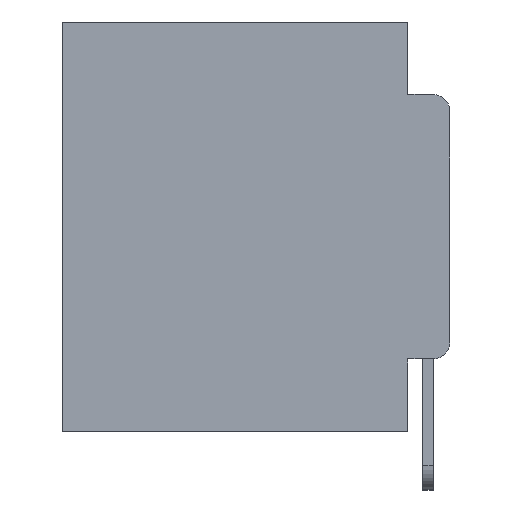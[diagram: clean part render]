
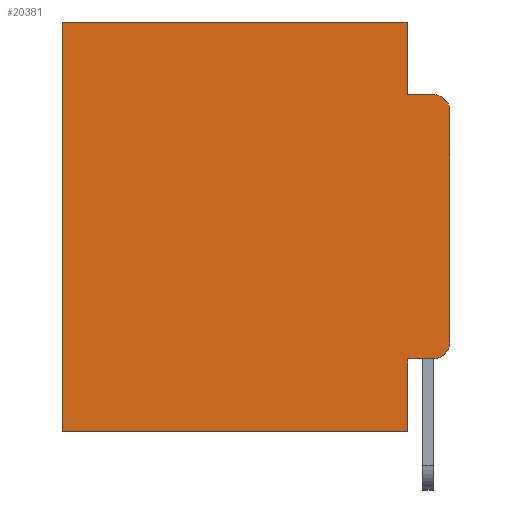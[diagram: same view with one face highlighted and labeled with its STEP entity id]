
A CAD part, left-side view. The second image highlights one B-rep face of the part: STEP entity #20381.
In plain terms, the highlighted planar face has unit normal (-1, 0, 0).
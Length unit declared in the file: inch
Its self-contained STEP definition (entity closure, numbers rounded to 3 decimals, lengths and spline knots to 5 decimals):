
#599 = VERTEX_POINT ( 'NONE', #14311 ) ;
#816 = VECTOR ( 'NONE', #19525, 39.37008 ) ;
#961 = CIRCLE ( 'NONE', #5620, 0.02 ) ;
#1031 = CARTESIAN_POINT ( 'NONE',  ( 0.298, 0., -0.5 ) ) ;
#1295 = DIRECTION ( 'NONE',  ( -1., 0., 0. ) ) ;
#1548 = AXIS2_PLACEMENT_3D ( 'NONE', #20681, #10157, #25126 ) ;
#1671 = CARTESIAN_POINT ( 'NONE',  ( 0.298, 0.051, 0. ) ) ;
#1893 = DIRECTION ( 'NONE',  ( 0., -1., 0. ) ) ;
#1897 = LINE ( 'NONE', #18239, #16613 ) ;
#2006 = LINE ( 'NONE', #21167, #19800 ) ;
#3149 = PLANE ( 'NONE',  #22982 ) ;
#3543 = LINE ( 'NONE', #19341, #816 ) ;
#3923 = EDGE_CURVE ( 'NONE', #20177, #22243, #6880, .T. ) ;
#4136 = VECTOR ( 'NONE', #6309, 39.37008 ) ;
#4221 = EDGE_CURVE ( 'NONE', #23742, #18434, #1897, .T. ) ;
#4287 = ORIENTED_EDGE ( 'NONE', *, *, #14657, .F. ) ;
#4483 = ORIENTED_EDGE ( 'NONE', *, *, #4221, .F. ) ;
#5059 = EDGE_CURVE ( 'NONE', #19185, #599, #14233, .T. ) ;
#5294 = DIRECTION ( 'NONE',  ( 0., 0., -1. ) ) ;
#5332 = DIRECTION ( 'NONE',  ( 0., 0., -1. ) ) ;
#5620 = AXIS2_PLACEMENT_3D ( 'NONE', #16380, #1295, #5332 ) ;
#6309 = DIRECTION ( 'NONE',  ( 0., 1., 0. ) ) ;
#6621 = CARTESIAN_POINT ( 'NONE',  ( 0.298, 0.473, 0. ) ) ;
#6880 = LINE ( 'NONE', #1671, #7564 ) ;
#7354 = FACE_OUTER_BOUND ( 'NONE', #10778, .T. ) ;
#7564 = VECTOR ( 'NONE', #12456, 39.37008 ) ;
#7922 = CIRCLE ( 'NONE', #1548, 0.02 ) ;
#8072 = CARTESIAN_POINT ( 'NONE',  ( 0.298, 0., -0.1085 ) ) ;
#8854 = VECTOR ( 'NONE', #9164, 39.37008 ) ;
#9157 = ORIENTED_EDGE ( 'NONE', *, *, #12754, .F. ) ;
#9164 = DIRECTION ( 'NONE',  ( 0., 0., -1. ) ) ;
#9547 = CARTESIAN_POINT ( 'NONE',  ( 0.298, 0.473, 0. ) ) ;
#10157 = DIRECTION ( 'NONE',  ( -1., 0., 0. ) ) ;
#10434 = VERTEX_POINT ( 'NONE', #8072 ) ;
#10778 = EDGE_LOOP ( 'NONE', ( #4287, #15771, #27266, #4483, #14500, #23023, #9157, #10780, #11809, #15659 ) ) ;
#10780 = ORIENTED_EDGE ( 'NONE', *, *, #3923, .F. ) ;
#11809 = ORIENTED_EDGE ( 'NONE', *, *, #18355, .T. ) ;
#11925 = CARTESIAN_POINT ( 'NONE',  ( 0.298, 0.051, -0.4115 ) ) ;
#12294 = VERTEX_POINT ( 'NONE', #17871 ) ;
#12456 = DIRECTION ( 'NONE',  ( 0., 0., -1. ) ) ;
#12754 = EDGE_CURVE ( 'NONE', #22243, #599, #23510, .T. ) ;
#13757 = CARTESIAN_POINT ( 'NONE',  ( 0.298, 0.02, -0.0885 ) ) ;
#13914 = DIRECTION ( 'NONE',  ( 0., 0., -1. ) ) ;
#14103 = CARTESIAN_POINT ( 'NONE',  ( 0.298, 0.051, -0.5 ) ) ;
#14233 = LINE ( 'NONE', #9547, #8854 ) ;
#14311 = CARTESIAN_POINT ( 'NONE',  ( 0.298, 0.473, -0.5 ) ) ;
#14441 = VERTEX_POINT ( 'NONE', #16406 ) ;
#14500 = ORIENTED_EDGE ( 'NONE', *, *, #16170, .T. ) ;
#14657 = EDGE_CURVE ( 'NONE', #10434, #14441, #3543, .T. ) ;
#15659 = ORIENTED_EDGE ( 'NONE', *, *, #22932, .T. ) ;
#15771 = ORIENTED_EDGE ( 'NONE', *, *, #18776, .T. ) ;
#16170 = EDGE_CURVE ( 'NONE', #23742, #19185, #16871, .T. ) ;
#16380 = CARTESIAN_POINT ( 'NONE',  ( 0.298, 0.02, -0.1085 ) ) ;
#16406 = CARTESIAN_POINT ( 'NONE',  ( 0.298, 0., -0.3915 ) ) ;
#16613 = VECTOR ( 'NONE', #5294, 39.37008 ) ;
#16871 = LINE ( 'NONE', #16974, #4136 ) ;
#16974 = CARTESIAN_POINT ( 'NONE',  ( 0.298, 0., 0. ) ) ;
#17205 = EDGE_CURVE ( 'NONE', #18434, #25533, #24944, .T. ) ;
#17255 = CARTESIAN_POINT ( 'NONE',  ( 0.298, 0.051, -0.0885 ) ) ;
#17395 = VECTOR ( 'NONE', #18205, 39.37008 ) ;
#17871 = CARTESIAN_POINT ( 'NONE',  ( 0.298, 0.02, -0.4115 ) ) ;
#18151 = DIRECTION ( 'NONE',  ( 1., 0., 0. ) ) ;
#18205 = DIRECTION ( 'NONE',  ( 0., 1., 0. ) ) ;
#18239 = CARTESIAN_POINT ( 'NONE',  ( 0.298, 0.051, 0. ) ) ;
#18355 = EDGE_CURVE ( 'NONE', #20177, #12294, #2006, .T. ) ;
#18434 = VERTEX_POINT ( 'NONE', #17255 ) ;
#18776 = EDGE_CURVE ( 'NONE', #10434, #25533, #961, .T. ) ;
#19185 = VERTEX_POINT ( 'NONE', #6621 ) ;
#19341 = CARTESIAN_POINT ( 'NONE',  ( 0.298, 0., 0. ) ) ;
#19525 = DIRECTION ( 'NONE',  ( 0., 0., -1. ) ) ;
#19800 = VECTOR ( 'NONE', #1893, 39.37008 ) ;
#19865 = DIRECTION ( 'NONE',  ( 0., -1., 0. ) ) ;
#20177 = VERTEX_POINT ( 'NONE', #11925 ) ;
#20381 = ADVANCED_FACE ( 'NONE', ( #7354 ), #3149, .F. ) ;
#20681 = CARTESIAN_POINT ( 'NONE',  ( 0.298, 0.02, -0.3915 ) ) ;
#21167 = CARTESIAN_POINT ( 'NONE',  ( 0.298, 0.051, -0.4115 ) ) ;
#22145 = CARTESIAN_POINT ( 'NONE',  ( 0.298, 0.051, -0.0885 ) ) ;
#22243 = VERTEX_POINT ( 'NONE', #14103 ) ;
#22932 = EDGE_CURVE ( 'NONE', #12294, #14441, #7922, .T. ) ;
#22982 = AXIS2_PLACEMENT_3D ( 'NONE', #26545, #18151, #13914 ) ;
#23023 = ORIENTED_EDGE ( 'NONE', *, *, #5059, .T. ) ;
#23252 = VECTOR ( 'NONE', #19865, 39.37008 ) ;
#23510 = LINE ( 'NONE', #1031, #17395 ) ;
#23742 = VERTEX_POINT ( 'NONE', #24719 ) ;
#24719 = CARTESIAN_POINT ( 'NONE',  ( 0.298, 0.051, 0. ) ) ;
#24944 = LINE ( 'NONE', #22145, #23252 ) ;
#25126 = DIRECTION ( 'NONE',  ( 0., 0., -1. ) ) ;
#25533 = VERTEX_POINT ( 'NONE', #13757 ) ;
#26545 = CARTESIAN_POINT ( 'NONE',  ( 0.298, 0., 0. ) ) ;
#27266 = ORIENTED_EDGE ( 'NONE', *, *, #17205, .F. ) ;
